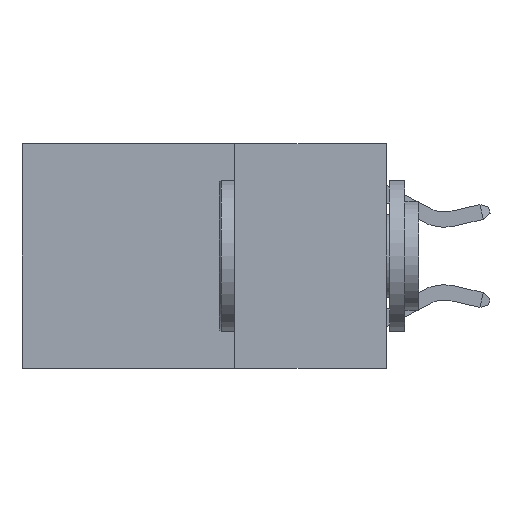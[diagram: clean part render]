
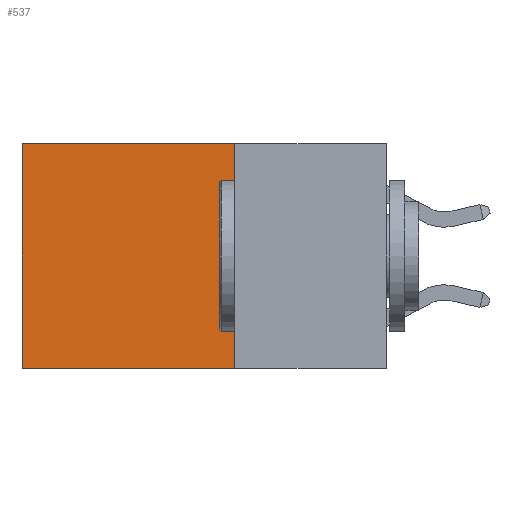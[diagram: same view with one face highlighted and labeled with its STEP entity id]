
A CAD part, left-side view. The second image highlights one B-rep face of the part: STEP entity #537.
In plain terms, the highlighted planar face has unit normal (-1, 0, 0).
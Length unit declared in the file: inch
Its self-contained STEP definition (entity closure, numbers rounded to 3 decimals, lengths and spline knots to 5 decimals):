
#63 = VECTOR ( 'NONE', #15937, 39.37008 ) ;
#69 = FACE_OUTER_BOUND ( 'NONE', #2130, .T. ) ;
#537 = ADVANCED_FACE ( 'NONE', ( #69 ), #28781, .F. ) ;
#901 = VECTOR ( 'NONE', #10470, 39.37008 ) ;
#1833 = EDGE_CURVE ( 'NONE', #8995, #11713, #27170, .T. ) ;
#1980 = EDGE_CURVE ( 'NONE', #11713, #12428, #8912, .T. ) ;
#2130 = EDGE_LOOP ( 'NONE', ( #7050, #26992, #28558, #15911 ) ) ;
#3130 = CARTESIAN_POINT ( 'NONE',  ( 0.2625, 0.25, 0. ) ) ;
#3592 = VECTOR ( 'NONE', #4428, 39.37008 ) ;
#4428 = DIRECTION ( 'NONE',  ( 0., 1., 0. ) ) ;
#7050 = ORIENTED_EDGE ( 'NONE', *, *, #1980, .T. ) ;
#8697 = CARTESIAN_POINT ( 'NONE',  ( 0.2625, 0.6, 0. ) ) ;
#8912 = LINE ( 'NONE', #27790, #63 ) ;
#8995 = VERTEX_POINT ( 'NONE', #20056 ) ;
#9747 = DIRECTION ( 'NONE',  ( 0., 0., -1. ) ) ;
#10470 = DIRECTION ( 'NONE',  ( 0., 0., -1. ) ) ;
#10956 = CARTESIAN_POINT ( 'NONE',  ( 0.2625, 0.25, 0. ) ) ;
#11713 = VERTEX_POINT ( 'NONE', #8697 ) ;
#12428 = VERTEX_POINT ( 'NONE', #19380 ) ;
#15327 = DIRECTION ( 'NONE',  ( 0., 1., 0. ) ) ;
#15911 = ORIENTED_EDGE ( 'NONE', *, *, #1833, .T. ) ;
#15937 = DIRECTION ( 'NONE',  ( 0., 0., -1. ) ) ;
#16682 = AXIS2_PLACEMENT_3D ( 'NONE', #24117, #26285, #9747 ) ;
#16719 = CARTESIAN_POINT ( 'NONE',  ( 0.2625, 0.25, -0.37 ) ) ;
#18621 = CARTESIAN_POINT ( 'NONE',  ( 0.2625, 0.25, -0.37 ) ) ;
#19380 = CARTESIAN_POINT ( 'NONE',  ( 0.2625, 0.6, -0.37 ) ) ;
#19485 = VERTEX_POINT ( 'NONE', #16719 ) ;
#20056 = CARTESIAN_POINT ( 'NONE',  ( 0.2625, 0.25, 0. ) ) ;
#22011 = VECTOR ( 'NONE', #15327, 39.37008 ) ;
#24117 = CARTESIAN_POINT ( 'NONE',  ( 0.2625, 0.25, 0. ) ) ;
#24528 = LINE ( 'NONE', #3130, #901 ) ;
#24621 = EDGE_CURVE ( 'NONE', #8995, #19485, #24528, .T. ) ;
#25360 = LINE ( 'NONE', #18621, #3592 ) ;
#26285 = DIRECTION ( 'NONE',  ( 1., 0., 0. ) ) ;
#26992 = ORIENTED_EDGE ( 'NONE', *, *, #28552, .F. ) ;
#27170 = LINE ( 'NONE', #10956, #22011 ) ;
#27790 = CARTESIAN_POINT ( 'NONE',  ( 0.2625, 0.6, 0. ) ) ;
#28552 = EDGE_CURVE ( 'NONE', #19485, #12428, #25360, .T. ) ;
#28558 = ORIENTED_EDGE ( 'NONE', *, *, #24621, .F. ) ;
#28781 = PLANE ( 'NONE',  #16682 ) ;
